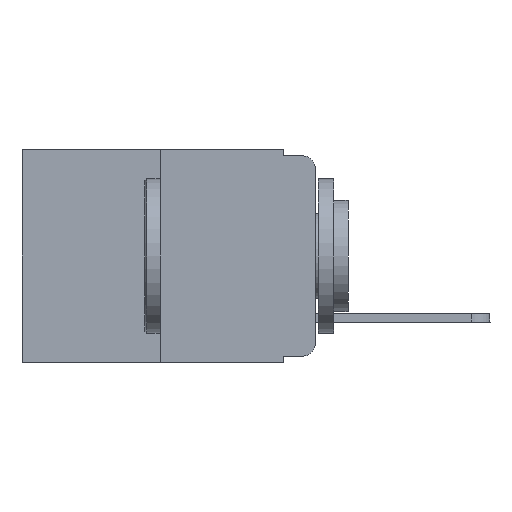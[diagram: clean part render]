
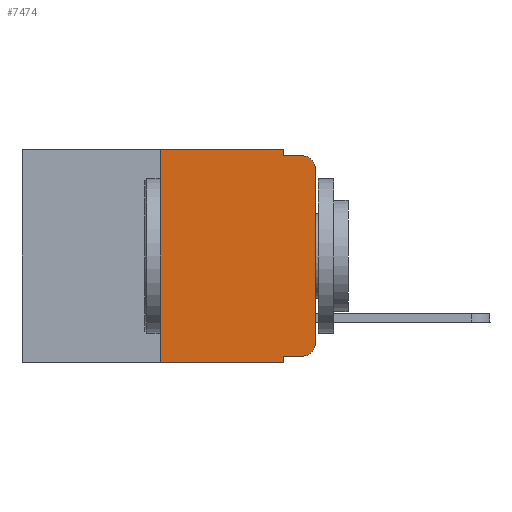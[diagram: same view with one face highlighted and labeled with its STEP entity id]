
A CAD part, left-side view. The second image highlights one B-rep face of the part: STEP entity #7474.
In plain terms, the highlighted planar face has unit normal (-1, 0, 0).
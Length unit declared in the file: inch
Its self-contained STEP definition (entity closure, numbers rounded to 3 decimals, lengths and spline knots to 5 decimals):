
#418 = LINE ( 'NONE', #8049, #17076 ) ;
#449 = LINE ( 'NONE', #12300, #12309 ) ;
#654 = AXIS2_PLACEMENT_3D ( 'NONE', #14403, #16980, #7792 ) ;
#870 = DIRECTION ( 'NONE',  ( 0., 0., -1. ) ) ;
#1168 = VECTOR ( 'NONE', #870, 39.37008 ) ;
#1443 = LINE ( 'NONE', #4362, #7040 ) ;
#1568 = LINE ( 'NONE', #16631, #1168 ) ;
#1915 = DIRECTION ( 'NONE',  ( 1., 0., 0. ) ) ;
#2497 = EDGE_CURVE ( 'NONE', #7765, #14327, #13936, .T. ) ;
#2595 = DIRECTION ( 'NONE',  ( 0., -1., 0. ) ) ;
#3124 = CARTESIAN_POINT ( 'NONE',  ( 0., 0.051, -0.343 ) ) ;
#3453 = ORIENTED_EDGE ( 'NONE', *, *, #14542, .F. ) ;
#3505 = CARTESIAN_POINT ( 'NONE',  ( 0., 0.02, -0.03 ) ) ;
#3604 = CARTESIAN_POINT ( 'NONE',  ( 0., 0.02, -0.333 ) ) ;
#3705 = VERTEX_POINT ( 'NONE', #3124 ) ;
#4002 = DIRECTION ( 'NONE',  ( 0., 0., -1. ) ) ;
#4032 = ORIENTED_EDGE ( 'NONE', *, *, #6416, .T. ) ;
#4337 = EDGE_CURVE ( 'NONE', #13748, #7932, #4933, .T. ) ;
#4362 = CARTESIAN_POINT ( 'NONE',  ( 0., 0.25, 0. ) ) ;
#4933 = LINE ( 'NONE', #14266, #9335 ) ;
#5432 = CARTESIAN_POINT ( 'NONE',  ( 0., 0.25, 0. ) ) ;
#5695 = ORIENTED_EDGE ( 'NONE', *, *, #2497, .F. ) ;
#5725 = ORIENTED_EDGE ( 'NONE', *, *, #9543, .F. ) ;
#5998 = CARTESIAN_POINT ( 'NONE',  ( 0., 0.051, -0.01 ) ) ;
#6117 = DIRECTION ( 'NONE',  ( -1., 0., 0. ) ) ;
#6322 = CARTESIAN_POINT ( 'NONE',  ( 0., 0.051, -0.333 ) ) ;
#6334 = PLANE ( 'NONE',  #10687 ) ;
#6378 = VERTEX_POINT ( 'NONE', #3604 ) ;
#6405 = VERTEX_POINT ( 'NONE', #5432 ) ;
#6416 = EDGE_CURVE ( 'NONE', #14342, #6378, #16232, .T. ) ;
#6571 = CARTESIAN_POINT ( 'NONE',  ( 0., 0.051, 0. ) ) ;
#7040 = VECTOR ( 'NONE', #13793, 39.37008 ) ;
#7260 = EDGE_CURVE ( 'NONE', #13038, #6405, #1443, .T. ) ;
#7474 = ADVANCED_FACE ( 'NONE', ( #12650 ), #6334, .F. ) ;
#7570 = VERTEX_POINT ( 'NONE', #6571 ) ;
#7765 = VERTEX_POINT ( 'NONE', #5998 ) ;
#7792 = DIRECTION ( 'NONE',  ( 0., 0., -1. ) ) ;
#7932 = VERTEX_POINT ( 'NONE', #10924 ) ;
#8049 = CARTESIAN_POINT ( 'NONE',  ( 0., 0.051, 0. ) ) ;
#8607 = ORIENTED_EDGE ( 'NONE', *, *, #7260, .F. ) ;
#8809 = EDGE_CURVE ( 'NONE', #7932, #14327, #12178, .T. ) ;
#8875 = ORIENTED_EDGE ( 'NONE', *, *, #9658, .T. ) ;
#9010 = ORIENTED_EDGE ( 'NONE', *, *, #8809, .T. ) ;
#9195 = VECTOR ( 'NONE', #2595, 39.37008 ) ;
#9335 = VECTOR ( 'NONE', #11668, 39.37008 ) ;
#9543 = EDGE_CURVE ( 'NONE', #14342, #3705, #1568, .T. ) ;
#9658 = EDGE_CURVE ( 'NONE', #6378, #13748, #10747, .T. ) ;
#9683 = VECTOR ( 'NONE', #9761, 39.37008 ) ;
#9761 = DIRECTION ( 'NONE',  ( 0., -1., 0. ) ) ;
#9905 = CARTESIAN_POINT ( 'NONE',  ( 0., 0.473, 0. ) ) ;
#10167 = DIRECTION ( 'NONE',  ( 0., 0., -1. ) ) ;
#10172 = AXIS2_PLACEMENT_3D ( 'NONE', #3505, #6117, #10167 ) ;
#10432 = CARTESIAN_POINT ( 'NONE',  ( 0., 0.02, -0.01 ) ) ;
#10687 = AXIS2_PLACEMENT_3D ( 'NONE', #9905, #1915, #15605 ) ;
#10747 = CIRCLE ( 'NONE', #654, 0.02 ) ;
#10924 = CARTESIAN_POINT ( 'NONE',  ( 0., 0., -0.03 ) ) ;
#11329 = CARTESIAN_POINT ( 'NONE',  ( 0., 0.051, -0.01 ) ) ;
#11450 = ORIENTED_EDGE ( 'NONE', *, *, #4337, .T. ) ;
#11668 = DIRECTION ( 'NONE',  ( 0., 0., 1. ) ) ;
#11846 = ORIENTED_EDGE ( 'NONE', *, *, #16605, .T. ) ;
#12178 = CIRCLE ( 'NONE', #10172, 0.02 ) ;
#12300 = CARTESIAN_POINT ( 'NONE',  ( 0., 0.473, -0.343 ) ) ;
#12309 = VECTOR ( 'NONE', #14709, 39.37008 ) ;
#12320 = CARTESIAN_POINT ( 'NONE',  ( 0., 0.25, -0.343 ) ) ;
#12650 = FACE_OUTER_BOUND ( 'NONE', #14581, .T. ) ;
#12652 = DIRECTION ( 'NONE',  ( 0., -1., 0. ) ) ;
#13038 = VERTEX_POINT ( 'NONE', #12320 ) ;
#13394 = LINE ( 'NONE', #15015, #9683 ) ;
#13748 = VERTEX_POINT ( 'NONE', #15661 ) ;
#13793 = DIRECTION ( 'NONE',  ( 0., 0., 1. ) ) ;
#13936 = LINE ( 'NONE', #11329, #16664 ) ;
#14266 = CARTESIAN_POINT ( 'NONE',  ( 0., 0., 0. ) ) ;
#14327 = VERTEX_POINT ( 'NONE', #10432 ) ;
#14342 = VERTEX_POINT ( 'NONE', #6322 ) ;
#14403 = CARTESIAN_POINT ( 'NONE',  ( 0., 0.02, -0.313 ) ) ;
#14542 = EDGE_CURVE ( 'NONE', #6405, #7570, #13394, .T. ) ;
#14581 = EDGE_LOOP ( 'NONE', ( #11450, #9010, #5695, #15974, #3453, #8607, #11846, #5725, #4032, #8875 ) ) ;
#14709 = DIRECTION ( 'NONE',  ( 0., -1., 0. ) ) ;
#15015 = CARTESIAN_POINT ( 'NONE',  ( 0., 0.473, 0. ) ) ;
#15605 = DIRECTION ( 'NONE',  ( 0., 0., -1. ) ) ;
#15661 = CARTESIAN_POINT ( 'NONE',  ( 0., 0., -0.313 ) ) ;
#15974 = ORIENTED_EDGE ( 'NONE', *, *, #17128, .F. ) ;
#15978 = CARTESIAN_POINT ( 'NONE',  ( 0., 0.051, -0.333 ) ) ;
#16232 = LINE ( 'NONE', #15978, #9195 ) ;
#16605 = EDGE_CURVE ( 'NONE', #13038, #3705, #449, .T. ) ;
#16631 = CARTESIAN_POINT ( 'NONE',  ( 0., 0.051, 0. ) ) ;
#16664 = VECTOR ( 'NONE', #12652, 39.37008 ) ;
#16980 = DIRECTION ( 'NONE',  ( -1., 0., 0. ) ) ;
#17076 = VECTOR ( 'NONE', #4002, 39.37008 ) ;
#17128 = EDGE_CURVE ( 'NONE', #7570, #7765, #418, .T. ) ;
